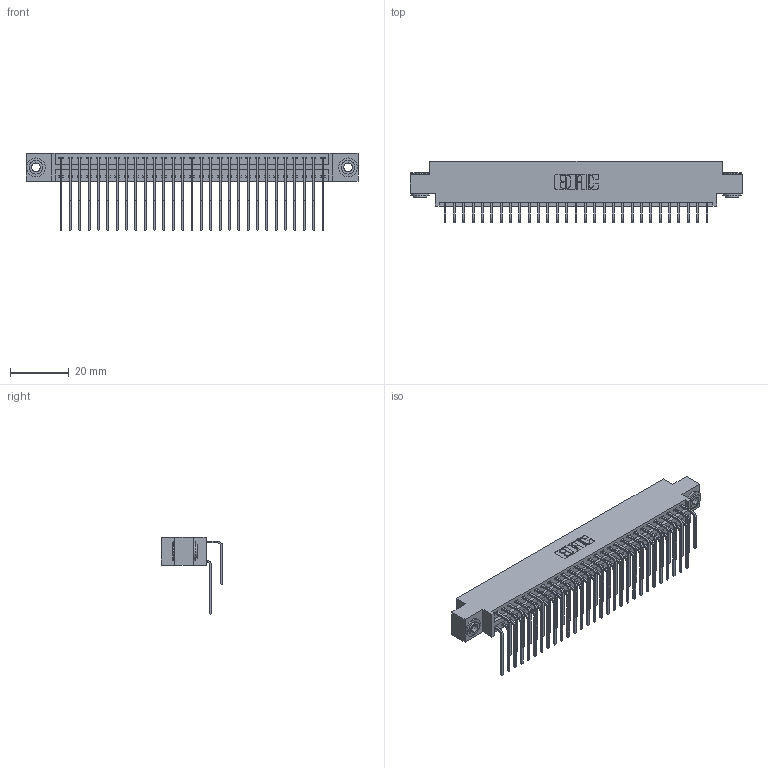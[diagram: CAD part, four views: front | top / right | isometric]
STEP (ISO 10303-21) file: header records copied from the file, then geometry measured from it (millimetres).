
FILE_DESCRIPTION (( 'STEP AP203' ), '1' );
FILE_NAME ('346-058-559-803.STEP', '2018-08-28T04:53:10', ( '' ), ( '' ), 'SwSTEP 2.0', 'SolidWorks 2016', '' );
FILE_SCHEMA (( 'CONFIG_CONTROL_DESIGN' ));
Length unit declared in the file: inch
Products named in the file (5): 346 Part_0.170 Offset - 0.156 Dia-TH; 345-292-001_558 559 Tail - 1; 345-292-001_559 Tail - 2; 345-250-002_345-250-002-102; 346-058-559-803
Assembly tree (61 placements, depth 2):
  346-058-559-803
    346 Part_0.170 Offset - 0.156 Dia-TH
    345-292-001_558 559 Tail - 1  x29
    345-292-001_559 Tail - 2  x29
    345-250-002_345-250-002-102  x2
Bounding box: 112.65 x 20.89 x 26.16 mm (x, y, z)
Volume: 11083.1 mm3; surface area: 17029 mm2
Topology: 61 solids, 61 shells, 3296 faces, 9755 edges, 6422 vertices
Faces by surface type: plane 2236, cylinder 1052, cone 8
Entity records: 23242 total; most frequent: CARTESIAN_POINT 3878, ORIENTED_EDGE 3754, DIRECTION 3471, EDGE_CURVE 1877, LINE 1565, VECTOR 1565, VERTEX_POINT 1246, AXIS2_PLACEMENT_3D 953
